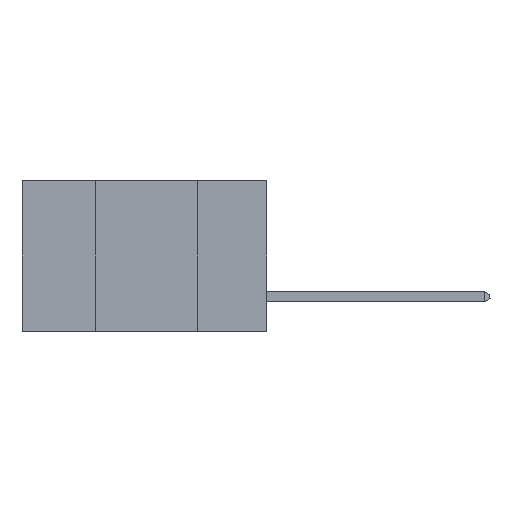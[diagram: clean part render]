
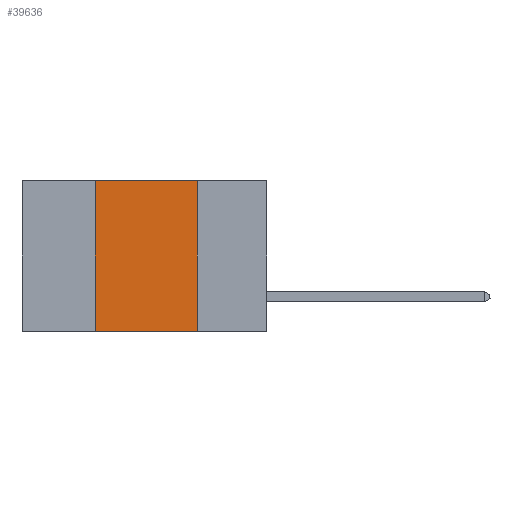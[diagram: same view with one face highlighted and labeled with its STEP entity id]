
A CAD part, left-side view. The second image highlights one B-rep face of the part: STEP entity #39636.
In plain terms, the highlighted planar face has unit normal (-1, 0, 0).
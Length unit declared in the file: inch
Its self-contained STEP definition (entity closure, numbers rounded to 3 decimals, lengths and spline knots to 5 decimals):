
#1735 = EDGE_LOOP ( 'NONE', ( #4097, #39246, #21380, #18140 ) ) ;
#2962 = VERTEX_POINT ( 'NONE', #4136 ) ;
#3122 = VECTOR ( 'NONE', #42716, 39.37008 ) ;
#4097 = ORIENTED_EDGE ( 'NONE', *, *, #29066, .F. ) ;
#4136 = CARTESIAN_POINT ( 'NONE',  ( 0., 0.42, -0.37 ) ) ;
#4681 = LINE ( 'NONE', #39323, #3122 ) ;
#4728 = VERTEX_POINT ( 'NONE', #15389 ) ;
#4774 = LINE ( 'NONE', #37235, #13176 ) ;
#7285 = EDGE_CURVE ( 'NONE', #2962, #31157, #40926, .T. ) ;
#8039 = CARTESIAN_POINT ( 'NONE',  ( 0., 0.17, 0. ) ) ;
#10381 = CARTESIAN_POINT ( 'NONE',  ( 0., 0.42, 0. ) ) ;
#11397 = DIRECTION ( 'NONE',  ( 0., 0., -1. ) ) ;
#11749 = FACE_OUTER_BOUND ( 'NONE', #1735, .T. ) ;
#13176 = VECTOR ( 'NONE', #24066, 39.37008 ) ;
#15389 = CARTESIAN_POINT ( 'NONE',  ( 0., 0.17, 0. ) ) ;
#16978 = CARTESIAN_POINT ( 'NONE',  ( 0., 0.42, 0. ) ) ;
#17109 = LINE ( 'NONE', #8039, #33897 ) ;
#17335 = VERTEX_POINT ( 'NONE', #23202 ) ;
#18140 = ORIENTED_EDGE ( 'NONE', *, *, #18835, .T. ) ;
#18835 = EDGE_CURVE ( 'NONE', #2962, #17335, #4774, .T. ) ;
#19703 = DIRECTION ( 'NONE',  ( 1., 0., 0. ) ) ;
#19985 = DIRECTION ( 'NONE',  ( 0., 0., -1. ) ) ;
#20978 = VECTOR ( 'NONE', #24446, 39.37008 ) ;
#21380 = ORIENTED_EDGE ( 'NONE', *, *, #7285, .F. ) ;
#22771 = EDGE_CURVE ( 'NONE', #31157, #4728, #4681, .T. ) ;
#23202 = CARTESIAN_POINT ( 'NONE',  ( 0., 0.17, -0.37 ) ) ;
#24066 = DIRECTION ( 'NONE',  ( 0., -1., 0. ) ) ;
#24446 = DIRECTION ( 'NONE',  ( 0., 0., 1. ) ) ;
#26160 = CARTESIAN_POINT ( 'NONE',  ( 0., 0.6, 0. ) ) ;
#29066 = EDGE_CURVE ( 'NONE', #4728, #17335, #17109, .T. ) ;
#31157 = VERTEX_POINT ( 'NONE', #16978 ) ;
#33897 = VECTOR ( 'NONE', #11397, 39.37008 ) ;
#36409 = PLANE ( 'NONE',  #41563 ) ;
#37235 = CARTESIAN_POINT ( 'NONE',  ( 0., 0.6, -0.37 ) ) ;
#39246 = ORIENTED_EDGE ( 'NONE', *, *, #22771, .F. ) ;
#39323 = CARTESIAN_POINT ( 'NONE',  ( 0., 0.6, 0. ) ) ;
#39636 = ADVANCED_FACE ( 'NONE', ( #11749 ), #36409, .F. ) ;
#40926 = LINE ( 'NONE', #10381, #20978 ) ;
#41563 = AXIS2_PLACEMENT_3D ( 'NONE', #26160, #19703, #19985 ) ;
#42716 = DIRECTION ( 'NONE',  ( 0., -1., 0. ) ) ;
